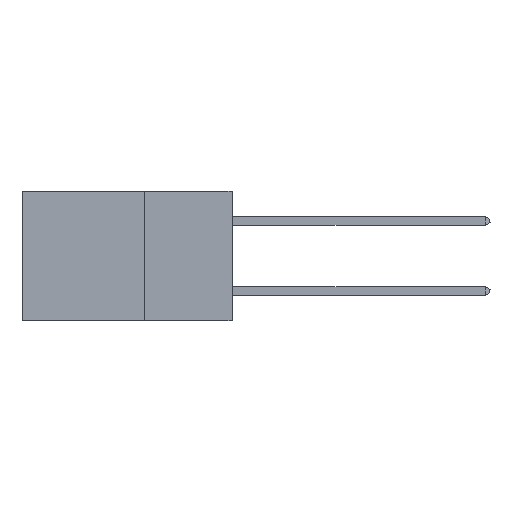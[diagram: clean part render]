
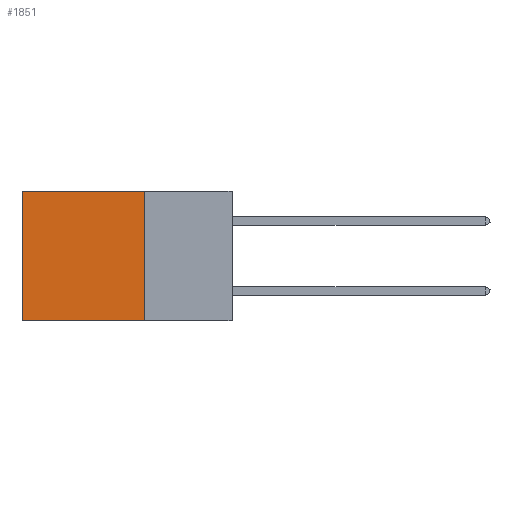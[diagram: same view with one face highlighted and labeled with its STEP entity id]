
A CAD part, left-side view. The second image highlights one B-rep face of the part: STEP entity #1851.
In plain terms, the highlighted planar face has unit normal (-1, 0, 0).
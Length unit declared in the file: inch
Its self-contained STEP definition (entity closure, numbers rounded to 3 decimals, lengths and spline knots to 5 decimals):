
#690 = CARTESIAN_POINT ( 'NONE',  ( 0.2875, 0.25, 0. ) ) ;
#1851 = ADVANCED_FACE ( 'NONE', ( #35259 ), #9898, .F. ) ;
#1873 = LINE ( 'NONE', #12107, #20139 ) ;
#3913 = EDGE_CURVE ( 'NONE', #25688, #23370, #5304, .T. ) ;
#4287 = EDGE_CURVE ( 'NONE', #29609, #23370, #1873, .T. ) ;
#5151 = LINE ( 'NONE', #27783, #31125 ) ;
#5304 = LINE ( 'NONE', #32595, #16751 ) ;
#6136 = DIRECTION ( 'NONE',  ( 0., 1., 0. ) ) ;
#6362 = CARTESIAN_POINT ( 'NONE',  ( 0.2875, 0.6, -0.37 ) ) ;
#9305 = CARTESIAN_POINT ( 'NONE',  ( 0.2875, 0.25, -0.37 ) ) ;
#9898 = PLANE ( 'NONE',  #32863 ) ;
#12098 = EDGE_LOOP ( 'NONE', ( #24902, #20925, #18219, #20612 ) ) ;
#12107 = CARTESIAN_POINT ( 'NONE',  ( 0.2875, 0.6, 0. ) ) ;
#15165 = DIRECTION ( 'NONE',  ( 0., 0., -1. ) ) ;
#15240 = CARTESIAN_POINT ( 'NONE',  ( 0.2875, 0.25, 0. ) ) ;
#15373 = DIRECTION ( 'NONE',  ( 0., 0., -1. ) ) ;
#16751 = VECTOR ( 'NONE', #18631, 39.37008 ) ;
#18219 = ORIENTED_EDGE ( 'NONE', *, *, #26873, .F. ) ;
#18426 = CARTESIAN_POINT ( 'NONE',  ( 0.2875, 0.25, 0. ) ) ;
#18631 = DIRECTION ( 'NONE',  ( 0., 1., 0. ) ) ;
#20139 = VECTOR ( 'NONE', #15165, 39.37008 ) ;
#20612 = ORIENTED_EDGE ( 'NONE', *, *, #26611, .T. ) ;
#20925 = ORIENTED_EDGE ( 'NONE', *, *, #3913, .F. ) ;
#23370 = VERTEX_POINT ( 'NONE', #6362 ) ;
#24681 = VERTEX_POINT ( 'NONE', #690 ) ;
#24902 = ORIENTED_EDGE ( 'NONE', *, *, #4287, .T. ) ;
#25688 = VERTEX_POINT ( 'NONE', #9305 ) ;
#26461 = DIRECTION ( 'NONE',  ( 1., 0., 0. ) ) ;
#26611 = EDGE_CURVE ( 'NONE', #24681, #29609, #5151, .T. ) ;
#26873 = EDGE_CURVE ( 'NONE', #24681, #25688, #31951, .T. ) ;
#27552 = CARTESIAN_POINT ( 'NONE',  ( 0.2875, 0.6, 0. ) ) ;
#27783 = CARTESIAN_POINT ( 'NONE',  ( 0.2875, 0.25, 0. ) ) ;
#28840 = DIRECTION ( 'NONE',  ( 0., 0., -1. ) ) ;
#29609 = VERTEX_POINT ( 'NONE', #27552 ) ;
#31125 = VECTOR ( 'NONE', #6136, 39.37008 ) ;
#31951 = LINE ( 'NONE', #15240, #33676 ) ;
#32595 = CARTESIAN_POINT ( 'NONE',  ( 0.2875, 0.25, -0.37 ) ) ;
#32863 = AXIS2_PLACEMENT_3D ( 'NONE', #18426, #26461, #28840 ) ;
#33676 = VECTOR ( 'NONE', #15373, 39.37008 ) ;
#35259 = FACE_OUTER_BOUND ( 'NONE', #12098, .T. ) ;
